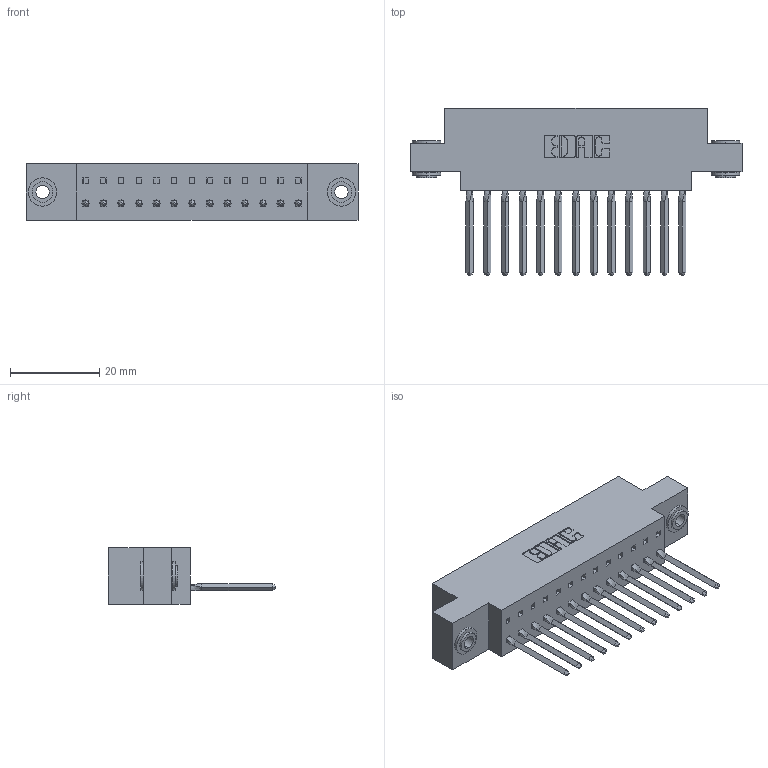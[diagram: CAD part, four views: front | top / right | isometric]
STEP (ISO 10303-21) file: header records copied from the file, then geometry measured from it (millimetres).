
FILE_DESCRIPTION (( 'STEP AP203' ), '1' );
FILE_NAME ('317-013-541-603.STEP', '2020-02-27T14:25:37', ( '' ), ( '' ), 'SwSTEP 2.0', 'SolidWorks 2016', '' );
FILE_SCHEMA (( 'CONFIG_CONTROL_DESIGN' ));
Length unit declared in the file: inch
Products named in the file (4): 317-013-541-603; 317 Part_.156 Dia - TH; 317-290-002_541; 345-250-002_345-250-002-102
Assembly tree (16 placements, depth 2):
  317-013-541-603
    317 Part_.156 Dia - TH
    317-290-002_541  x13
    345-250-002_345-250-002-102  x2
Bounding box: 74.22 x 37.34 x 12.7 mm (x, y, z)
Volume: 11163.5 mm3; surface area: 15022.6 mm2
Topology: 16 solids, 16 shells, 2116 faces, 5993 edges, 3896 vertices
Faces by surface type: plane 1680, cylinder 376, bspline 52, cone 8
Entity records: 24619 total; most frequent: CARTESIAN_POINT 4971, ORIENTED_EDGE 4230, DIRECTION 3495, EDGE_CURVE 2115, VECTOR 1727, LINE 1727, VERTEX_POINT 1400, AXIS2_PLACEMENT_3D 884
